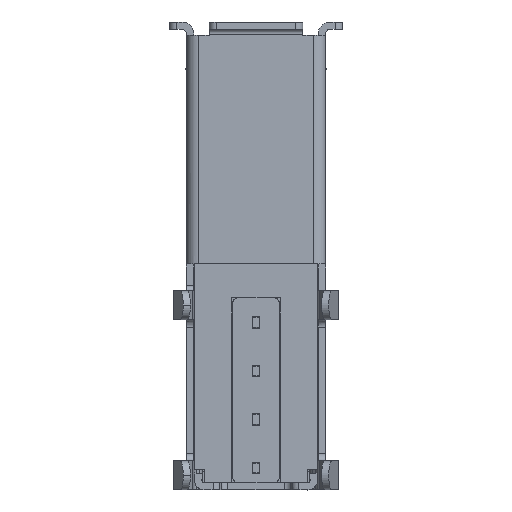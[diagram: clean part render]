
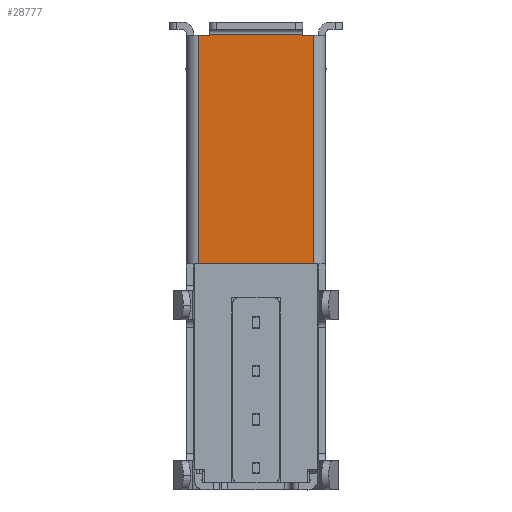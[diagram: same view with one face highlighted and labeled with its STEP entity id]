
A CAD part, front view. The second image highlights one B-rep face of the part: STEP entity #28777.
In plain terms, the highlighted planar face has unit normal (0, -1, 0).
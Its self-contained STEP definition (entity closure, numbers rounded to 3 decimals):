
#1021 = VERTEX_POINT ( 'NONE', #33762 ) ;
#1089 = LINE ( 'NONE', #28893, #11595 ) ;
#1980 = CARTESIAN_POINT ( 'NONE',  ( -3.305, -6.55, -1.925 ) ) ;
#2026 = ORIENTED_EDGE ( 'NONE', *, *, #35433, .T. ) ;
#2387 = EDGE_CURVE ( 'NONE', #17045, #8453, #30811, .T. ) ;
#2651 = CARTESIAN_POINT ( 'NONE',  ( -8.518, -6.55, 2.36 ) ) ;
#2707 = CARTESIAN_POINT ( 'NONE',  ( -8.33, -6.55, 0.88 ) ) ;
#2760 = ORIENTED_EDGE ( 'NONE', *, *, #33365, .F. ) ;
#3061 = VERTEX_POINT ( 'NONE', #21505 ) ;
#3163 = ORIENTED_EDGE ( 'NONE', *, *, #7124, .F. ) ;
#3391 = EDGE_CURVE ( 'NONE', #14639, #38445, #8059, .T. ) ;
#4101 = VECTOR ( 'NONE', #14191, 1000. ) ;
#4287 = CARTESIAN_POINT ( 'NONE',  ( 1.52, -6.55, 0.75 ) ) ;
#4664 = VERTEX_POINT ( 'NONE', #20282 ) ;
#4818 = CARTESIAN_POINT ( 'NONE',  ( -8.33, -6.55, -0.88 ) ) ;
#6065 = VECTOR ( 'NONE', #13765, 1000. ) ;
#6323 = LINE ( 'NONE', #18659, #22653 ) ;
#6616 = VECTOR ( 'NONE', #26964, 1000. ) ;
#7124 = EDGE_CURVE ( 'NONE', #8145, #17045, #26341, .T. ) ;
#7550 = ORIENTED_EDGE ( 'NONE', *, *, #24760, .F. ) ;
#7682 = CARTESIAN_POINT ( 'NONE',  ( 1.77, -6.55, -0.88 ) ) ;
#7812 = CARTESIAN_POINT ( 'NONE',  ( -8.518, -6.55, -2.36 ) ) ;
#8059 = CIRCLE ( 'NONE', #26500, 0.25 ) ;
#8145 = VERTEX_POINT ( 'NONE', #36970 ) ;
#8326 = VERTEX_POINT ( 'NONE', #38322 ) ;
#8453 = VERTEX_POINT ( 'NONE', #36873 ) ;
#8694 = VECTOR ( 'NONE', #35989, 1000. ) ;
#8947 = VECTOR ( 'NONE', #32494, 1000. ) ;
#9409 = CARTESIAN_POINT ( 'NONE',  ( -3.305, -6.55, -0.88 ) ) ;
#9860 = AXIS2_PLACEMENT_3D ( 'NONE', #4287, #33918, #16229 ) ;
#9947 = CARTESIAN_POINT ( 'NONE',  ( 1.07, -6.55, -2.36 ) ) ;
#10244 = CARTESIAN_POINT ( 'NONE',  ( 1.52, -6.55, 1. ) ) ;
#10379 = LINE ( 'NONE', #22512, #22680 ) ;
#10637 = CARTESIAN_POINT ( 'NONE',  ( -8.33, -6.55, -1.925 ) ) ;
#10800 = ORIENTED_EDGE ( 'NONE', *, *, #38738, .F. ) ;
#11595 = VECTOR ( 'NONE', #19184, 1000. ) ;
#11884 = VECTOR ( 'NONE', #31750, 1000. ) ;
#11986 = DIRECTION ( 'NONE',  ( 1., 0., 0. ) ) ;
#12527 = CARTESIAN_POINT ( 'NONE',  ( 1.07, -6.55, 0.88 ) ) ;
#12782 = FACE_OUTER_BOUND ( 'NONE', #38526, .T. ) ;
#13566 = AXIS2_PLACEMENT_3D ( 'NONE', #9409, #27900, #30878 ) ;
#13623 = EDGE_CURVE ( 'NONE', #21842, #37545, #27695, .T. ) ;
#13765 = DIRECTION ( 'NONE',  ( 0., 0., 1. ) ) ;
#13867 = CARTESIAN_POINT ( 'NONE',  ( 1.77, -6.55, -0.75 ) ) ;
#14191 = DIRECTION ( 'NONE',  ( -1., 0., 0. ) ) ;
#14527 = LINE ( 'NONE', #1980, #8694 ) ;
#14639 = VERTEX_POINT ( 'NONE', #13867 ) ;
#14981 = CARTESIAN_POINT ( 'NONE',  ( -8.33, -6.55, 2.36 ) ) ;
#16229 = DIRECTION ( 'NONE',  ( 0., 0., -1. ) ) ;
#17045 = VERTEX_POINT ( 'NONE', #10244 ) ;
#17156 = VERTEX_POINT ( 'NONE', #10637 ) ;
#17173 = LINE ( 'NONE', #7812, #4101 ) ;
#17208 = CARTESIAN_POINT ( 'NONE',  ( -3.305, -6.55, 1. ) ) ;
#17502 = DIRECTION ( 'NONE',  ( 0., 1., 0. ) ) ;
#18659 = CARTESIAN_POINT ( 'NONE',  ( -3.305, -6.55, 1.925 ) ) ;
#18762 = PLANE ( 'NONE',  #13566 ) ;
#18914 = EDGE_CURVE ( 'NONE', #38445, #1021, #1089, .T. ) ;
#19064 = ORIENTED_EDGE ( 'NONE', *, *, #13623, .F. ) ;
#19079 = DIRECTION ( 'NONE',  ( 0., 0., -1. ) ) ;
#19184 = DIRECTION ( 'NONE',  ( -1., 0., 0. ) ) ;
#19543 = DIRECTION ( 'NONE',  ( 0., 0., 1. ) ) ;
#19650 = LINE ( 'NONE', #25398, #11884 ) ;
#20282 = CARTESIAN_POINT ( 'NONE',  ( -8.38, -6.55, 1.925 ) ) ;
#20476 = CARTESIAN_POINT ( 'NONE',  ( 1.52, -6.55, -0.75 ) ) ;
#20822 = VERTEX_POINT ( 'NONE', #9947 ) ;
#21469 = CARTESIAN_POINT ( 'NONE',  ( -8.33, -6.55, 1.925 ) ) ;
#21505 = CARTESIAN_POINT ( 'NONE',  ( -8.33, -6.55, -2.36 ) ) ;
#21842 = VERTEX_POINT ( 'NONE', #14981 ) ;
#22284 = ORIENTED_EDGE ( 'NONE', *, *, #3391, .F. ) ;
#22512 = CARTESIAN_POINT ( 'NONE',  ( -8.38, -6.55, -0.88 ) ) ;
#22653 = VECTOR ( 'NONE', #30574, 1000. ) ;
#22680 = VECTOR ( 'NONE', #19543, 1000. ) ;
#22709 = EDGE_CURVE ( 'NONE', #4664, #35293, #6323, .T. ) ;
#22841 = ORIENTED_EDGE ( 'NONE', *, *, #30844, .F. ) ;
#22872 = ORIENTED_EDGE ( 'NONE', *, *, #35076, .F. ) ;
#23102 = VECTOR ( 'NONE', #19079, 1000. ) ;
#24760 = EDGE_CURVE ( 'NONE', #8326, #4664, #10379, .T. ) ;
#25398 = CARTESIAN_POINT ( 'NONE',  ( 1.07, -6.55, 0. ) ) ;
#25478 = LINE ( 'NONE', #4818, #6065 ) ;
#26341 = LINE ( 'NONE', #17208, #8947 ) ;
#26500 = AXIS2_PLACEMENT_3D ( 'NONE', #20476, #17502, #35776 ) ;
#26957 = CARTESIAN_POINT ( 'NONE',  ( 1.07, -6.55, 2.36 ) ) ;
#26964 = DIRECTION ( 'NONE',  ( 0., 0., 1. ) ) ;
#27350 = LINE ( 'NONE', #2707, #6616 ) ;
#27695 = LINE ( 'NONE', #2651, #37525 ) ;
#27900 = DIRECTION ( 'NONE',  ( 0., 1., 0. ) ) ;
#28265 = ORIENTED_EDGE ( 'NONE', *, *, #22709, .F. ) ;
#28777 = ADVANCED_FACE ( 'NONE', ( #12782 ), #18762, .F. ) ;
#28893 = CARTESIAN_POINT ( 'NONE',  ( -3.305, -6.55, -1. ) ) ;
#30574 = DIRECTION ( 'NONE',  ( 1., 0., 0. ) ) ;
#30635 = VECTOR ( 'NONE', #38299, 1000. ) ;
#30811 = CIRCLE ( 'NONE', #9860, 0.25 ) ;
#30844 = EDGE_CURVE ( 'NONE', #8453, #14639, #35133, .T. ) ;
#30878 = DIRECTION ( 'NONE',  ( 0., 0., 1. ) ) ;
#31750 = DIRECTION ( 'NONE',  ( 0., 0., 1. ) ) ;
#32494 = DIRECTION ( 'NONE',  ( 1., 0., 0. ) ) ;
#33365 = EDGE_CURVE ( 'NONE', #3061, #17156, #25478, .T. ) ;
#33756 = CARTESIAN_POINT ( 'NONE',  ( 1.52, -6.55, -1. ) ) ;
#33762 = CARTESIAN_POINT ( 'NONE',  ( 1.07, -6.55, -1. ) ) ;
#33918 = DIRECTION ( 'NONE',  ( 0., 1., 0. ) ) ;
#34372 = LINE ( 'NONE', #12527, #23102 ) ;
#35076 = EDGE_CURVE ( 'NONE', #17156, #8326, #14527, .T. ) ;
#35133 = LINE ( 'NONE', #7682, #30635 ) ;
#35274 = ORIENTED_EDGE ( 'NONE', *, *, #18914, .F. ) ;
#35293 = VERTEX_POINT ( 'NONE', #21469 ) ;
#35433 = EDGE_CURVE ( 'NONE', #20822, #1021, #19650, .T. ) ;
#35776 = DIRECTION ( 'NONE',  ( 0., 0., -1. ) ) ;
#35869 = ORIENTED_EDGE ( 'NONE', *, *, #39028, .F. ) ;
#35989 = DIRECTION ( 'NONE',  ( -1., 0., 0. ) ) ;
#36030 = ORIENTED_EDGE ( 'NONE', *, *, #2387, .F. ) ;
#36873 = CARTESIAN_POINT ( 'NONE',  ( 1.77, -6.55, 0.75 ) ) ;
#36891 = EDGE_CURVE ( 'NONE', #37545, #8145, #34372, .T. ) ;
#36970 = CARTESIAN_POINT ( 'NONE',  ( 1.07, -6.55, 1. ) ) ;
#37525 = VECTOR ( 'NONE', #11986, 1000. ) ;
#37545 = VERTEX_POINT ( 'NONE', #26957 ) ;
#38299 = DIRECTION ( 'NONE',  ( 0., 0., -1. ) ) ;
#38322 = CARTESIAN_POINT ( 'NONE',  ( -8.38, -6.55, -1.925 ) ) ;
#38341 = ORIENTED_EDGE ( 'NONE', *, *, #36891, .F. ) ;
#38445 = VERTEX_POINT ( 'NONE', #33756 ) ;
#38526 = EDGE_LOOP ( 'NONE', ( #35274, #22284, #22841, #36030, #3163, #38341, #19064, #10800, #28265, #7550, #22872, #2760, #35869, #2026 ) ) ;
#38738 = EDGE_CURVE ( 'NONE', #35293, #21842, #27350, .T. ) ;
#39028 = EDGE_CURVE ( 'NONE', #20822, #3061, #17173, .T. ) ;
